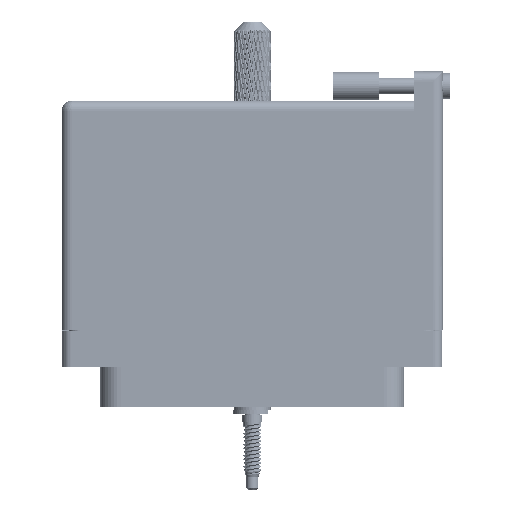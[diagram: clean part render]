
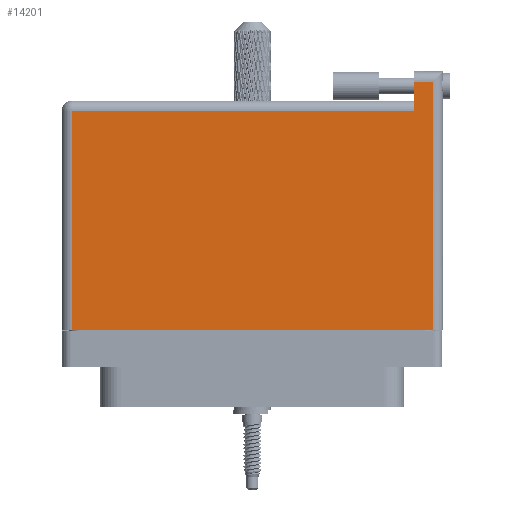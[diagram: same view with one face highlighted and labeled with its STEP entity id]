
A CAD part, front view. The second image highlights one B-rep face of the part: STEP entity #14201.
In plain terms, the highlighted face is planar.
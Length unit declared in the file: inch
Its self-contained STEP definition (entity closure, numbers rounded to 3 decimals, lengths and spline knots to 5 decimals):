
#295 = LINE ( 'NONE', #98053, #18744 ) ;
#447 = VECTOR ( 'NONE', #27289, 39.37008 ) ;
#811 = VERTEX_POINT ( 'NONE', #81365 ) ;
#1240 = EDGE_CURVE ( 'NONE', #29334, #17192, #72784, .T. ) ;
#5511 = DIRECTION ( 'NONE',  ( 1., 0., 0. ) ) ;
#12106 = DIRECTION ( 'NONE',  ( 0., 1., 0. ) ) ;
#14201 = ADVANCED_FACE ( 'NONE', ( #73512 ), #114602, .F. ) ;
#14230 = DIRECTION ( 'NONE',  ( 0., 0., -1. ) ) ;
#17192 = VERTEX_POINT ( 'NONE', #17267 ) ;
#17267 = CARTESIAN_POINT ( 'NONE',  ( 1.23, -0.1, 0.4495 ) ) ;
#18744 = VECTOR ( 'NONE', #78709, 39.37008 ) ;
#19333 = CARTESIAN_POINT ( 'NONE',  ( -1.3, 1.396, 0.4495 ) ) ;
#19336 = ORIENTED_EDGE ( 'NONE', *, *, #65476, .T. ) ;
#21617 = ORIENTED_EDGE ( 'NONE', *, *, #81115, .T. ) ;
#21655 = EDGE_CURVE ( 'NONE', #67667, #811, #80648, .T. ) ;
#27289 = DIRECTION ( 'NONE',  ( -1., 0., 0. ) ) ;
#29334 = VERTEX_POINT ( 'NONE', #71345 ) ;
#34989 = VECTOR ( 'NONE', #12106, 39.37008 ) ;
#36431 = EDGE_LOOP ( 'NONE', ( #114469, #19336, #116576, #106562, #21617, #52510 ) ) ;
#40433 = CARTESIAN_POINT ( 'NONE',  ( -1.3, 1.466, 0.4495 ) ) ;
#42108 = CARTESIAN_POINT ( 'NONE',  ( -1.23, 1.396, 0.4495 ) ) ;
#46053 = EDGE_CURVE ( 'NONE', #811, #83103, #295, .T. ) ;
#49165 = AXIS2_PLACEMENT_3D ( 'NONE', #40433, #14230, #96034 ) ;
#49936 = CARTESIAN_POINT ( 'NONE',  ( -1.3, -0.1, 0.4495 ) ) ;
#51615 = DIRECTION ( 'NONE',  ( 0., -1., 0. ) ) ;
#52510 = ORIENTED_EDGE ( 'NONE', *, *, #76953, .T. ) ;
#54352 = VECTOR ( 'NONE', #5511, 39.37008 ) ;
#55853 = CARTESIAN_POINT ( 'NONE',  ( -1.3, 1.596, 0.4495 ) ) ;
#63044 = DIRECTION ( 'NONE',  ( -1., 0., 0. ) ) ;
#65476 = EDGE_CURVE ( 'NONE', #17192, #67667, #82024, .T. ) ;
#67667 = VERTEX_POINT ( 'NONE', #74477 ) ;
#68768 = CARTESIAN_POINT ( 'NONE',  ( -1.23, -0.1, 0.4495 ) ) ;
#71345 = CARTESIAN_POINT ( 'NONE',  ( -1.23, -0.1, 0.4495 ) ) ;
#72784 = LINE ( 'NONE', #49936, #54352 ) ;
#73512 = FACE_OUTER_BOUND ( 'NONE', #36431, .T. ) ;
#74477 = CARTESIAN_POINT ( 'NONE',  ( 1.23, 1.596, 0.4495 ) ) ;
#76953 = EDGE_CURVE ( 'NONE', #111879, #29334, #91345, .T. ) ;
#78709 = DIRECTION ( 'NONE',  ( 0., -1., 0. ) ) ;
#80648 = LINE ( 'NONE', #55853, #101842 ) ;
#81115 = EDGE_CURVE ( 'NONE', #83103, #111879, #85657, .T. ) ;
#81365 = CARTESIAN_POINT ( 'NONE',  ( 1.103, 1.596, 0.4495 ) ) ;
#82024 = LINE ( 'NONE', #85515, #34989 ) ;
#83103 = VERTEX_POINT ( 'NONE', #115647 ) ;
#85515 = CARTESIAN_POINT ( 'NONE',  ( 1.23, 1.666, 0.4495 ) ) ;
#85657 = LINE ( 'NONE', #19333, #447 ) ;
#91345 = LINE ( 'NONE', #68768, #99849 ) ;
#96034 = DIRECTION ( 'NONE',  ( -1., 0., 0. ) ) ;
#98053 = CARTESIAN_POINT ( 'NONE',  ( 1.103, 1.666, 0.4495 ) ) ;
#99849 = VECTOR ( 'NONE', #51615, 39.37008 ) ;
#101842 = VECTOR ( 'NONE', #63044, 39.37008 ) ;
#106562 = ORIENTED_EDGE ( 'NONE', *, *, #46053, .T. ) ;
#111879 = VERTEX_POINT ( 'NONE', #42108 ) ;
#114469 = ORIENTED_EDGE ( 'NONE', *, *, #1240, .T. ) ;
#114602 = PLANE ( 'NONE',  #49165 ) ;
#115647 = CARTESIAN_POINT ( 'NONE',  ( 1.103, 1.396, 0.4495 ) ) ;
#116576 = ORIENTED_EDGE ( 'NONE', *, *, #21655, .T. ) ;
